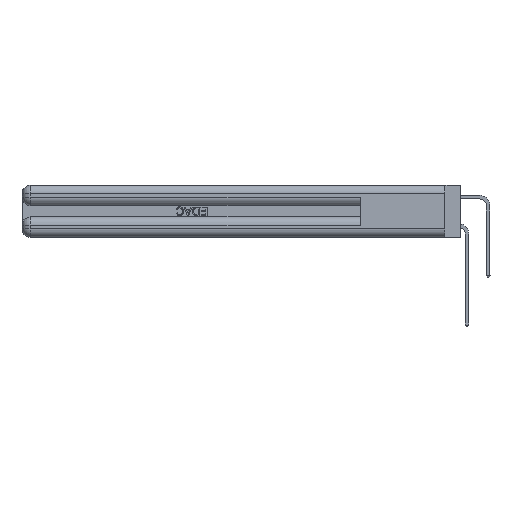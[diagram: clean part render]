
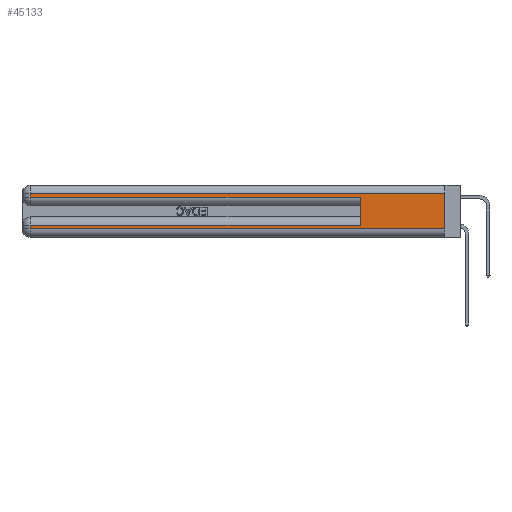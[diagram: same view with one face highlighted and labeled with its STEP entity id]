
A CAD part, left-side view. The second image highlights one B-rep face of the part: STEP entity #45133.
In plain terms, the highlighted planar face has unit normal (-1, 0, 0).
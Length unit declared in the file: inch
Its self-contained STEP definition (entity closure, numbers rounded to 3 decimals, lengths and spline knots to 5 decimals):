
#541 = VECTOR ( 'NONE', #31477, 39.37008 ) ;
#800 = VERTEX_POINT ( 'NONE', #5101 ) ;
#1245 = PLANE ( 'NONE',  #15591 ) ;
#1412 = VECTOR ( 'NONE', #41966, 39.37008 ) ;
#1956 = VERTEX_POINT ( 'NONE', #47749 ) ;
#2401 = EDGE_LOOP ( 'NONE', ( #5908, #20881, #16151, #30308, #29316, #6591, #12442, #43713 ) ) ;
#2517 = EDGE_CURVE ( 'NONE', #800, #14512, #24366, .T. ) ;
#3313 = VECTOR ( 'NONE', #15792, 39.37008 ) ;
#5101 = CARTESIAN_POINT ( 'NONE',  ( 0., 2.94, 0.06 ) ) ;
#5263 = EDGE_CURVE ( 'NONE', #33752, #1956, #28330, .T. ) ;
#5908 = ORIENTED_EDGE ( 'NONE', *, *, #16053, .F. ) ;
#6591 = ORIENTED_EDGE ( 'NONE', *, *, #38661, .T. ) ;
#6658 = VECTOR ( 'NONE', #26008, 39.37008 ) ;
#7304 = CARTESIAN_POINT ( 'NONE',  ( 0., 0.6, 0.145 ) ) ;
#7881 = CARTESIAN_POINT ( 'NONE',  ( 0., 0., 0.06 ) ) ;
#8688 = VERTEX_POINT ( 'NONE', #24124 ) ;
#10901 = CARTESIAN_POINT ( 'NONE',  ( 0., 0., 0.285 ) ) ;
#11770 = CARTESIAN_POINT ( 'NONE',  ( 0., 2.94, 0.37 ) ) ;
#12442 = ORIENTED_EDGE ( 'NONE', *, *, #32320, .T. ) ;
#13072 = CARTESIAN_POINT ( 'NONE',  ( 0., 0., 0.31 ) ) ;
#13257 = LINE ( 'NONE', #18462, #6658 ) ;
#13401 = LINE ( 'NONE', #30689, #30134 ) ;
#13538 = LINE ( 'NONE', #11770, #3313 ) ;
#14512 = VERTEX_POINT ( 'NONE', #36364 ) ;
#15434 = DIRECTION ( 'NONE',  ( 0., -1., 0. ) ) ;
#15591 = AXIS2_PLACEMENT_3D ( 'NONE', #24706, #28072, #32405 ) ;
#15792 = DIRECTION ( 'NONE',  ( 0., 0., -1. ) ) ;
#16053 = EDGE_CURVE ( 'NONE', #44752, #14512, #13257, .T. ) ;
#16151 = ORIENTED_EDGE ( 'NONE', *, *, #39948, .T. ) ;
#16176 = LINE ( 'NONE', #13072, #541 ) ;
#18462 = CARTESIAN_POINT ( 'NONE',  ( 0., 0., 0.37 ) ) ;
#18998 = CARTESIAN_POINT ( 'NONE',  ( 0., 2.94, 0.31 ) ) ;
#20702 = EDGE_CURVE ( 'NONE', #33281, #1956, #30152, .T. ) ;
#20881 = ORIENTED_EDGE ( 'NONE', *, *, #30137, .T. ) ;
#22571 = DIRECTION ( 'NONE',  ( 0., 1., 0. ) ) ;
#24124 = CARTESIAN_POINT ( 'NONE',  ( 0., 2.94, 0.085 ) ) ;
#24366 = LINE ( 'NONE', #7881, #41708 ) ;
#24706 = CARTESIAN_POINT ( 'NONE',  ( 0., 0., 0.37 ) ) ;
#25215 = CARTESIAN_POINT ( 'NONE',  ( 0., 0.6, 0.085 ) ) ;
#25788 = DIRECTION ( 'NONE',  ( 0., -1., 0. ) ) ;
#26008 = DIRECTION ( 'NONE',  ( 0., 0., -1. ) ) ;
#28072 = DIRECTION ( 'NONE',  ( 1., 0., 0. ) ) ;
#28330 = LINE ( 'NONE', #10901, #45720 ) ;
#28879 = VERTEX_POINT ( 'NONE', #18998 ) ;
#29316 = ORIENTED_EDGE ( 'NONE', *, *, #20702, .F. ) ;
#30134 = VECTOR ( 'NONE', #37899, 39.37008 ) ;
#30137 = EDGE_CURVE ( 'NONE', #44752, #28879, #16176, .T. ) ;
#30152 = LINE ( 'NONE', #7304, #1412 ) ;
#30308 = ORIENTED_EDGE ( 'NONE', *, *, #5263, .T. ) ;
#30689 = CARTESIAN_POINT ( 'NONE',  ( 0., 2.94, 0.37 ) ) ;
#31273 = FACE_OUTER_BOUND ( 'NONE', #2401, .T. ) ;
#31477 = DIRECTION ( 'NONE',  ( 0., 1., 0. ) ) ;
#31500 = LINE ( 'NONE', #42026, #32696 ) ;
#32320 = EDGE_CURVE ( 'NONE', #8688, #800, #13538, .T. ) ;
#32405 = DIRECTION ( 'NONE',  ( 0., 0., -1. ) ) ;
#32696 = VECTOR ( 'NONE', #22571, 39.37008 ) ;
#33281 = VERTEX_POINT ( 'NONE', #25215 ) ;
#33752 = VERTEX_POINT ( 'NONE', #43944 ) ;
#36364 = CARTESIAN_POINT ( 'NONE',  ( 0., 0., 0.06 ) ) ;
#37899 = DIRECTION ( 'NONE',  ( 0., 0., -1. ) ) ;
#38661 = EDGE_CURVE ( 'NONE', #33281, #8688, #31500, .T. ) ;
#39948 = EDGE_CURVE ( 'NONE', #28879, #33752, #13401, .T. ) ;
#41646 = CARTESIAN_POINT ( 'NONE',  ( 0., 0., 0.31 ) ) ;
#41708 = VECTOR ( 'NONE', #15434, 39.37008 ) ;
#41966 = DIRECTION ( 'NONE',  ( 0., 0., 1. ) ) ;
#42026 = CARTESIAN_POINT ( 'NONE',  ( 0., 0., 0.085 ) ) ;
#43713 = ORIENTED_EDGE ( 'NONE', *, *, #2517, .T. ) ;
#43944 = CARTESIAN_POINT ( 'NONE',  ( 0., 2.94, 0.285 ) ) ;
#44752 = VERTEX_POINT ( 'NONE', #41646 ) ;
#45133 = ADVANCED_FACE ( 'NONE', ( #31273 ), #1245, .F. ) ;
#45720 = VECTOR ( 'NONE', #25788, 39.37008 ) ;
#47749 = CARTESIAN_POINT ( 'NONE',  ( 0., 0.6, 0.285 ) ) ;
